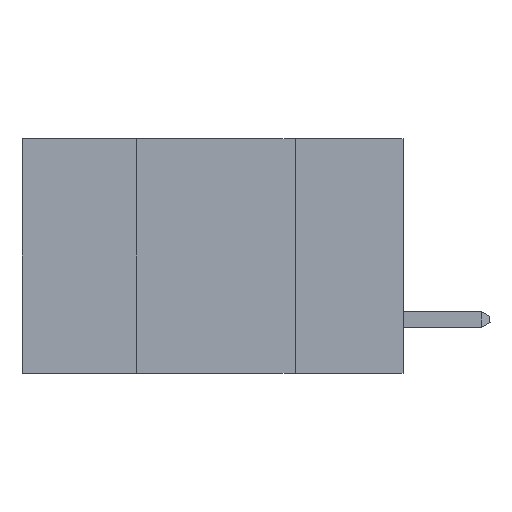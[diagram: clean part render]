
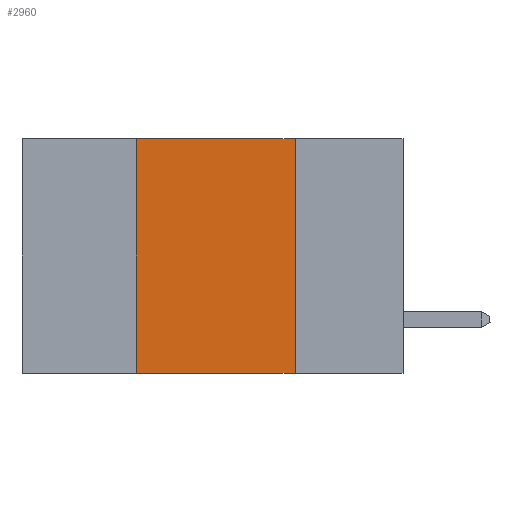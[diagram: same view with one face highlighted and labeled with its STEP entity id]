
A CAD part, left-side view. The second image highlights one B-rep face of the part: STEP entity #2960.
In plain terms, the highlighted planar face has unit normal (-1, 0, 0).
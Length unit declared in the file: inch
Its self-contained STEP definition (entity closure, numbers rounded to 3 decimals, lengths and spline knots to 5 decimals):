
#79 = LINE ( 'NONE', #3060, #2732 ) ;
#382 = LINE ( 'NONE', #7132, #8795 ) ;
#397 = CARTESIAN_POINT ( 'NONE',  ( 0., 0.42, -0.37 ) ) ;
#598 = DIRECTION ( 'NONE',  ( 0., 0., 1. ) ) ;
#672 = CARTESIAN_POINT ( 'NONE',  ( 0., 0.42, 0. ) ) ;
#692 = VERTEX_POINT ( 'NONE', #672 ) ;
#858 = PLANE ( 'NONE',  #7879 ) ;
#1936 = VERTEX_POINT ( 'NONE', #7963 ) ;
#1990 = ORIENTED_EDGE ( 'NONE', *, *, #3677, .F. ) ;
#2732 = VECTOR ( 'NONE', #6087, 39.37008 ) ;
#2940 = LINE ( 'NONE', #7240, #4886 ) ;
#2960 = ADVANCED_FACE ( 'NONE', ( #7996 ), #858, .F. ) ;
#3002 = VERTEX_POINT ( 'NONE', #9074 ) ;
#3060 = CARTESIAN_POINT ( 'NONE',  ( 0., 0.6, -0.37 ) ) ;
#3091 = ORIENTED_EDGE ( 'NONE', *, *, #3147, .F. ) ;
#3147 = EDGE_CURVE ( 'NONE', #3002, #1936, #382, .T. ) ;
#3230 = VECTOR ( 'NONE', #6310, 39.37008 ) ;
#3677 = EDGE_CURVE ( 'NONE', #692, #3002, #8440, .T. ) ;
#4140 = DIRECTION ( 'NONE',  ( 0., 0., -1. ) ) ;
#4202 = ORIENTED_EDGE ( 'NONE', *, *, #5645, .F. ) ;
#4886 = VECTOR ( 'NONE', #598, 39.37008 ) ;
#5161 = EDGE_CURVE ( 'NONE', #9285, #1936, #79, .T. ) ;
#5221 = CARTESIAN_POINT ( 'NONE',  ( 0., 0.6, 0. ) ) ;
#5645 = EDGE_CURVE ( 'NONE', #9285, #692, #2940, .T. ) ;
#6087 = DIRECTION ( 'NONE',  ( 0., -1., 0. ) ) ;
#6109 = ORIENTED_EDGE ( 'NONE', *, *, #5161, .T. ) ;
#6310 = DIRECTION ( 'NONE',  ( 0., -1., 0. ) ) ;
#6323 = EDGE_LOOP ( 'NONE', ( #3091, #1990, #4202, #6109 ) ) ;
#6378 = CARTESIAN_POINT ( 'NONE',  ( 0., 0.6, 0. ) ) ;
#7132 = CARTESIAN_POINT ( 'NONE',  ( 0., 0.17, 0. ) ) ;
#7240 = CARTESIAN_POINT ( 'NONE',  ( 0., 0.42, 0. ) ) ;
#7438 = DIRECTION ( 'NONE',  ( 0., 0., -1. ) ) ;
#7879 = AXIS2_PLACEMENT_3D ( 'NONE', #5221, #8984, #7438 ) ;
#7963 = CARTESIAN_POINT ( 'NONE',  ( 0., 0.17, -0.37 ) ) ;
#7996 = FACE_OUTER_BOUND ( 'NONE', #6323, .T. ) ;
#8440 = LINE ( 'NONE', #6378, #3230 ) ;
#8795 = VECTOR ( 'NONE', #4140, 39.37008 ) ;
#8984 = DIRECTION ( 'NONE',  ( 1., 0., 0. ) ) ;
#9074 = CARTESIAN_POINT ( 'NONE',  ( 0., 0.17, 0. ) ) ;
#9285 = VERTEX_POINT ( 'NONE', #397 ) ;
